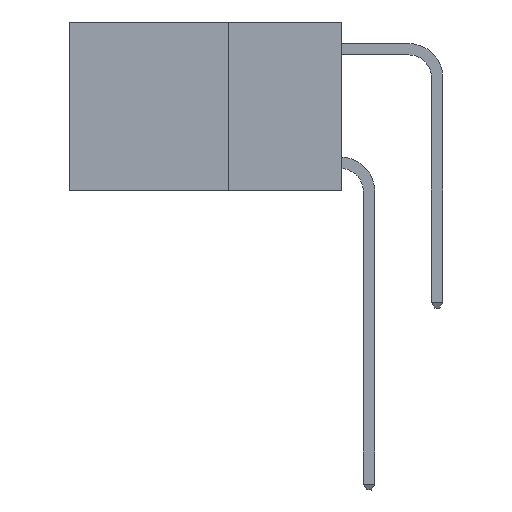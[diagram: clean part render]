
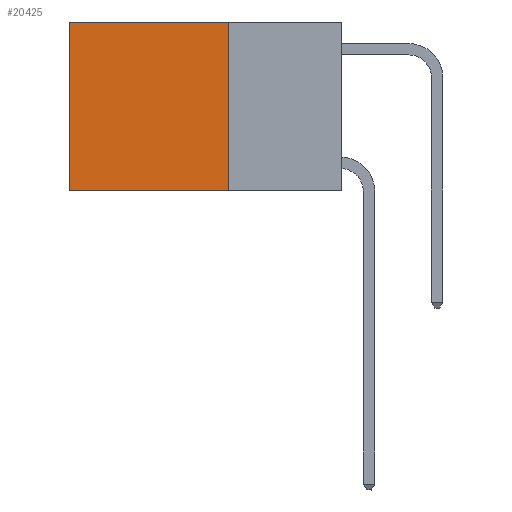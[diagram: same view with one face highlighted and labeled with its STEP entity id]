
A CAD part, left-side view. The second image highlights one B-rep face of the part: STEP entity #20425.
In plain terms, the highlighted planar face has unit normal (-1, 0, 0).
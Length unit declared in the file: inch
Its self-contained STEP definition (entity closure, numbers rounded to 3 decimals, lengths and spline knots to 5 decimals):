
#257 = ORIENTED_EDGE ( 'NONE', *, *, #1708, .F. ) ;
#629 = VECTOR ( 'NONE', #14220, 39.37008 ) ;
#1708 = EDGE_CURVE ( 'NONE', #3860, #10284, #7283, .T. ) ;
#3860 = VERTEX_POINT ( 'NONE', #3903 ) ;
#3903 = CARTESIAN_POINT ( 'NONE',  ( 0.2625, 0.25, -0.37 ) ) ;
#3979 = VECTOR ( 'NONE', #13216, 39.37008 ) ;
#5724 = CARTESIAN_POINT ( 'NONE',  ( 0.2625, 0.6, 0. ) ) ;
#6865 = CARTESIAN_POINT ( 'NONE',  ( 0.2625, 0.25, 0. ) ) ;
#7283 = LINE ( 'NONE', #10410, #23296 ) ;
#8235 = ORIENTED_EDGE ( 'NONE', *, *, #15206, .T. ) ;
#9088 = VERTEX_POINT ( 'NONE', #6865 ) ;
#9348 = CARTESIAN_POINT ( 'NONE',  ( 0.2625, 0.6, -0.37 ) ) ;
#9649 = LINE ( 'NONE', #21526, #3979 ) ;
#10173 = EDGE_CURVE ( 'NONE', #9088, #16161, #9649, .T. ) ;
#10284 = VERTEX_POINT ( 'NONE', #9348 ) ;
#10399 = CARTESIAN_POINT ( 'NONE',  ( 0.2625, 0.25, 0. ) ) ;
#10410 = CARTESIAN_POINT ( 'NONE',  ( 0.2625, 0.25, -0.37 ) ) ;
#11416 = CARTESIAN_POINT ( 'NONE',  ( 0.2625, 0.25, 0. ) ) ;
#11427 = LINE ( 'NONE', #11416, #21895 ) ;
#12516 = DIRECTION ( 'NONE',  ( 1., 0., 0. ) ) ;
#13216 = DIRECTION ( 'NONE',  ( 0., 1., 0. ) ) ;
#13542 = DIRECTION ( 'NONE',  ( 0., 0., -1. ) ) ;
#13970 = FACE_OUTER_BOUND ( 'NONE', #21803, .T. ) ;
#14220 = DIRECTION ( 'NONE',  ( 0., 0., -1. ) ) ;
#15206 = EDGE_CURVE ( 'NONE', #16161, #10284, #16894, .T. ) ;
#16161 = VERTEX_POINT ( 'NONE', #26413 ) ;
#16563 = AXIS2_PLACEMENT_3D ( 'NONE', #10399, #12516, #27016 ) ;
#16894 = LINE ( 'NONE', #5724, #629 ) ;
#17931 = EDGE_CURVE ( 'NONE', #9088, #3860, #11427, .T. ) ;
#20425 = ADVANCED_FACE ( 'NONE', ( #13970 ), #22908, .F. ) ;
#21526 = CARTESIAN_POINT ( 'NONE',  ( 0.2625, 0.25, 0. ) ) ;
#21803 = EDGE_LOOP ( 'NONE', ( #8235, #257, #23453, #23156 ) ) ;
#21895 = VECTOR ( 'NONE', #13542, 39.37008 ) ;
#22908 = PLANE ( 'NONE',  #16563 ) ;
#23156 = ORIENTED_EDGE ( 'NONE', *, *, #10173, .T. ) ;
#23296 = VECTOR ( 'NONE', #27029, 39.37008 ) ;
#23453 = ORIENTED_EDGE ( 'NONE', *, *, #17931, .F. ) ;
#26413 = CARTESIAN_POINT ( 'NONE',  ( 0.2625, 0.6, 0. ) ) ;
#27016 = DIRECTION ( 'NONE',  ( 0., 0., -1. ) ) ;
#27029 = DIRECTION ( 'NONE',  ( 0., 1., 0. ) ) ;
